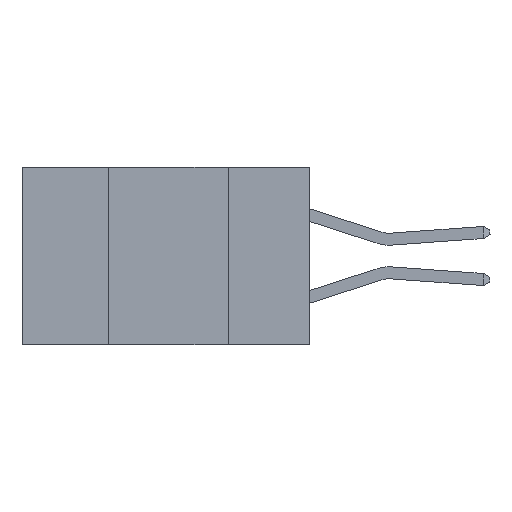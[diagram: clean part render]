
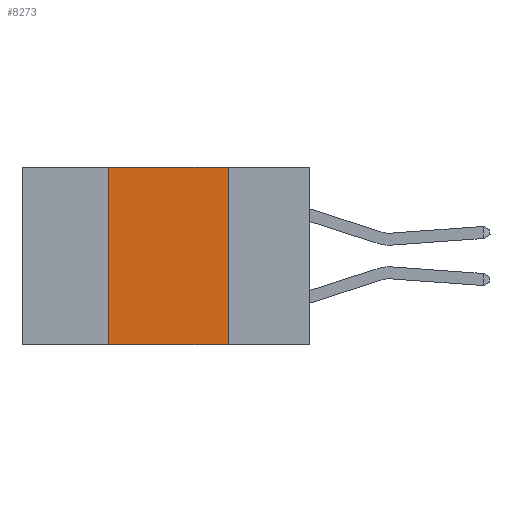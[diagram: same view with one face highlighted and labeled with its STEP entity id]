
A CAD part, left-side view. The second image highlights one B-rep face of the part: STEP entity #8273.
In plain terms, the highlighted planar face has unit normal (-1, 0, 0).
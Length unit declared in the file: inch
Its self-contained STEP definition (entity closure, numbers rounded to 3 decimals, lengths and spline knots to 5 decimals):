
#574 = VERTEX_POINT ( 'NONE', #13299 ) ;
#1079 = LINE ( 'NONE', #1191, #5831 ) ;
#1191 = CARTESIAN_POINT ( 'NONE',  ( 0., 0.42, -0.37 ) ) ;
#1204 = CARTESIAN_POINT ( 'NONE',  ( 0., 0.17, -0.37 ) ) ;
#2131 = EDGE_LOOP ( 'NONE', ( #14789, #15365, #18776, #17350 ) ) ;
#2410 = VERTEX_POINT ( 'NONE', #23771 ) ;
#2629 = LINE ( 'NONE', #17365, #18174 ) ;
#2950 = CARTESIAN_POINT ( 'NONE',  ( 0., 0.6, 0. ) ) ;
#2972 = EDGE_CURVE ( 'NONE', #3870, #574, #9371, .T. ) ;
#3870 = VERTEX_POINT ( 'NONE', #17894 ) ;
#4179 = EDGE_CURVE ( 'NONE', #3870, #5499, #1079, .T. ) ;
#4183 = VECTOR ( 'NONE', #14158, 39.37008 ) ;
#4345 = DIRECTION ( 'NONE',  ( 0., 0., 1. ) ) ;
#4620 = VECTOR ( 'NONE', #18545, 39.37008 ) ;
#4662 = EDGE_CURVE ( 'NONE', #5499, #2410, #2629, .T. ) ;
#5076 = LINE ( 'NONE', #1204, #4183 ) ;
#5499 = VERTEX_POINT ( 'NONE', #15826 ) ;
#5643 = CARTESIAN_POINT ( 'NONE',  ( 0., 0.6, -0.37 ) ) ;
#5831 = VECTOR ( 'NONE', #4345, 39.37008 ) ;
#6492 = DIRECTION ( 'NONE',  ( 0., -1., 0. ) ) ;
#8273 = ADVANCED_FACE ( 'NONE', ( #17694 ), #20620, .F. ) ;
#9371 = LINE ( 'NONE', #5643, #4620 ) ;
#13299 = CARTESIAN_POINT ( 'NONE',  ( 0., 0.17, -0.37 ) ) ;
#14158 = DIRECTION ( 'NONE',  ( 0., 0., -1. ) ) ;
#14789 = ORIENTED_EDGE ( 'NONE', *, *, #15160, .F. ) ;
#15160 = EDGE_CURVE ( 'NONE', #2410, #574, #5076, .T. ) ;
#15365 = ORIENTED_EDGE ( 'NONE', *, *, #4662, .F. ) ;
#15761 = DIRECTION ( 'NONE',  ( 1., 0., 0. ) ) ;
#15826 = CARTESIAN_POINT ( 'NONE',  ( 0., 0.42, 0. ) ) ;
#17350 = ORIENTED_EDGE ( 'NONE', *, *, #2972, .T. ) ;
#17365 = CARTESIAN_POINT ( 'NONE',  ( 0., 0.6, 0. ) ) ;
#17694 = FACE_OUTER_BOUND ( 'NONE', #2131, .T. ) ;
#17848 = AXIS2_PLACEMENT_3D ( 'NONE', #2950, #15761, #22547 ) ;
#17894 = CARTESIAN_POINT ( 'NONE',  ( 0., 0.42, -0.37 ) ) ;
#18174 = VECTOR ( 'NONE', #6492, 39.37008 ) ;
#18545 = DIRECTION ( 'NONE',  ( 0., -1., 0. ) ) ;
#18776 = ORIENTED_EDGE ( 'NONE', *, *, #4179, .F. ) ;
#20620 = PLANE ( 'NONE',  #17848 ) ;
#22547 = DIRECTION ( 'NONE',  ( 0., 0., -1. ) ) ;
#23771 = CARTESIAN_POINT ( 'NONE',  ( 0., 0.17, 0. ) ) ;
